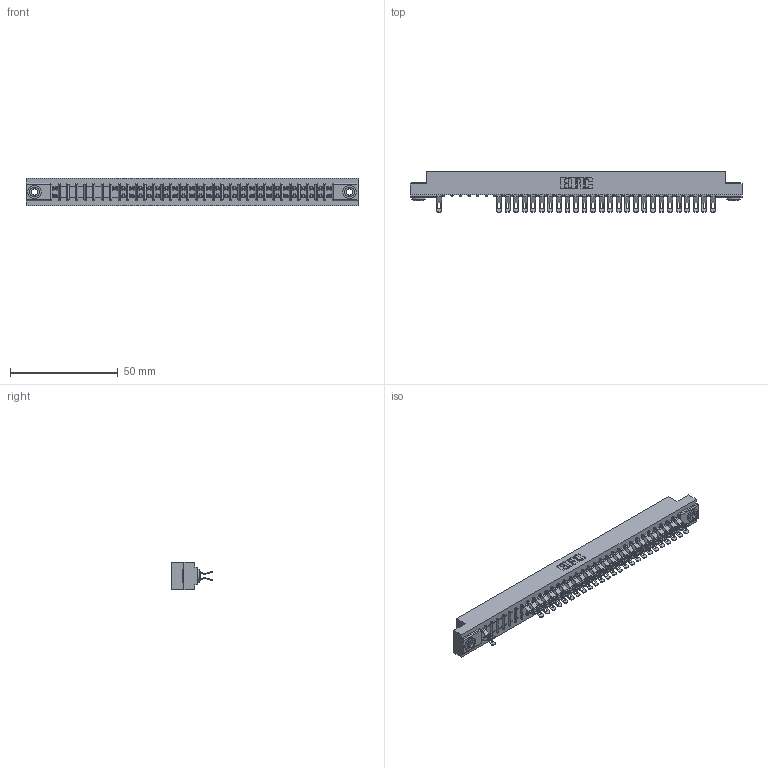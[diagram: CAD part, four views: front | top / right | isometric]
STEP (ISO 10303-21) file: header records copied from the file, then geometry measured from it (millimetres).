
FILE_DESCRIPTION (( 'STEP AP203' ), '1' );
FILE_NAME ('307-066-555-203.STEP', '2018-08-06T11:13:53', ( '' ), ( '' ), 'SwSTEP 2.0', 'SolidWorks 2016', '' );
FILE_SCHEMA (( 'CONFIG_CONTROL_DESIGN' ));
Length unit declared in the file: inch
Products named in the file (4): 307-066-555-203; 307 Part_.156 Dia Mounting Holes; 307-290-001_555; 345-250-002_345-250-002-102
Assembly tree (56 placements, depth 2):
  307-066-555-203
    307 Part_.156 Dia Mounting Holes
    307-290-001_555  x53
    345-250-002_345-250-002-102  x2
Bounding box: 153.77 x 18.75 x 12.7 mm (x, y, z)
Volume: 16278.9 mm3; surface area: 19758.2 mm2
Topology: 56 solids, 56 shells, 3567 faces, 10444 edges, 6796 vertices
Faces by surface type: plane 1974, cylinder 1517, sphere 68, cone 8
Entity records: 31642 total; most frequent: CARTESIAN_POINT 5221, ORIENTED_EDGE 5180, DIRECTION 5126, EDGE_CURVE 2590, LINE 1964, VECTOR 1964, VERTEX_POINT 1676, AXIS2_PLACEMENT_3D 1581
